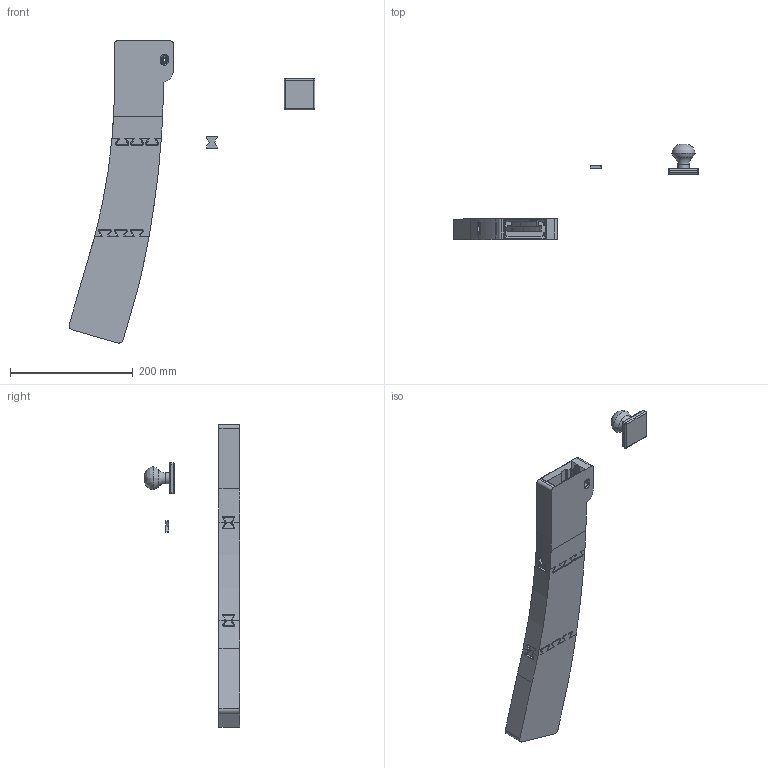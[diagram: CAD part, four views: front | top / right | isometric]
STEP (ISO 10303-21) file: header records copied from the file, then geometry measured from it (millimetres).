
FILE_DESCRIPTION(/* description */ (''),/* implementation_level */ '2;1');
FILE_NAME(/* name */ 'freeman1337-ar15-mag-speed-loader-all-v6-FINAL.step',/* time_stamp */ '2021-09-04T08:27:57-07:00',/* author */ (''),/* organization */ (''),/* preprocessor_version */ 'ST-DEVELOPER v18.1',/* originating_system */ 'Autodesk Translation Framework v10.10.0.1391',/* authorisation */ '');
FILE_SCHEMA (('AUTOMOTIVE_DESIGN { 1 0 10303 214 3 1 1 }'));
Products named in the file (1): (Unsaved)
Bounding box: 399.6 x 154.65 x 491.38 mm (x, y, z)
Volume: 838962.1 mm3; surface area: 187584.4 mm2
Topology: 5 solids, 6 shells, 4522 faces, 12306 edges, 8116 vertices
Faces by surface type: bspline 2856, plane 1379, cylinder 249, torus 23, sphere 9, cone 6
Full cylindrical faces by diameter (mm): 5.182 x1, 7.925 x1, 18 x1
Entity records: 156664 total; most frequent: CARTESIAN_POINT 66199, ORIENTED_EDGE 24602, EDGE_CURVE 12301, DIRECTION 11379, VERTEX_POINT 8116, LINE 6055, VECTOR 6055, EDGE_LOOP 4853
